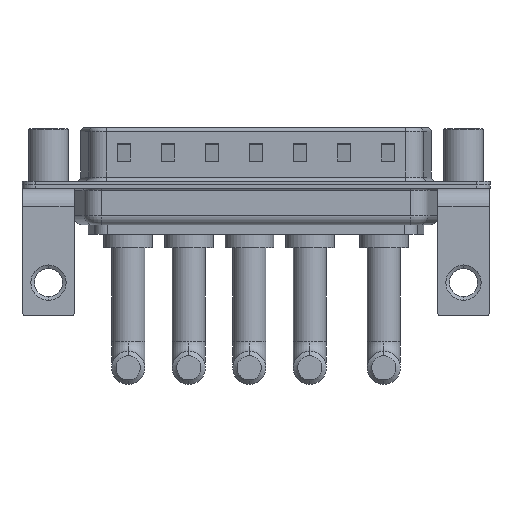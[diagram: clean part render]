
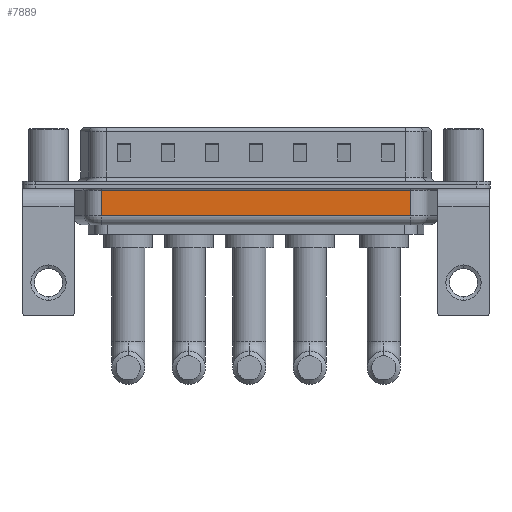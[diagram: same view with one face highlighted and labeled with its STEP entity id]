
A CAD part, front view. The second image highlights one B-rep face of the part: STEP entity #7889.
In plain terms, the highlighted planar face has unit normal (0, -1, 0).
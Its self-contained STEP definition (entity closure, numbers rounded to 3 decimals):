
#407 = EDGE_CURVE ( 'NONE', #15320, #16307, #5819, .T. ) ;
#557 = VECTOR ( 'NONE', #15797, 1000. ) ;
#854 = LINE ( 'NONE', #16324, #9173 ) ;
#1092 = PLANE ( 'NONE',  #11755 ) ;
#1909 = EDGE_LOOP ( 'NONE', ( #11771, #5399, #3220, #3569 ) ) ;
#2048 = CARTESIAN_POINT ( 'NONE',  ( 41.044, -5.35, -0.65 ) ) ;
#3220 = ORIENTED_EDGE ( 'NONE', *, *, #407, .T. ) ;
#3242 = DIRECTION ( 'NONE',  ( 0., 0., 1. ) ) ;
#3560 = VERTEX_POINT ( 'NONE', #6634 ) ;
#3569 = ORIENTED_EDGE ( 'NONE', *, *, #16784, .T. ) ;
#4444 = VERTEX_POINT ( 'NONE', #11022 ) ;
#5340 = CARTESIAN_POINT ( 'NONE',  ( 6.006, -5.35, -4.5 ) ) ;
#5399 = ORIENTED_EDGE ( 'NONE', *, *, #7920, .T. ) ;
#5819 = LINE ( 'NONE', #15003, #10045 ) ;
#6634 = CARTESIAN_POINT ( 'NONE',  ( 6.006, -5.35, -3.5 ) ) ;
#7732 = FACE_OUTER_BOUND ( 'NONE', #1909, .T. ) ;
#7889 = ADVANCED_FACE ( 'NONE', ( #7732 ), #1092, .F. ) ;
#7895 = DIRECTION ( 'NONE',  ( 0., 1., 0. ) ) ;
#7920 = EDGE_CURVE ( 'NONE', #3560, #15320, #9182, .T. ) ;
#9173 = VECTOR ( 'NONE', #11368, 1000. ) ;
#9182 = LINE ( 'NONE', #12974, #557 ) ;
#9682 = VECTOR ( 'NONE', #11806, 1000. ) ;
#9732 = CARTESIAN_POINT ( 'NONE',  ( 41.044, -5.35, -3.5 ) ) ;
#10045 = VECTOR ( 'NONE', #3242, 1000. ) ;
#11022 = CARTESIAN_POINT ( 'NONE',  ( 6.006, -5.35, -0.65 ) ) ;
#11368 = DIRECTION ( 'NONE',  ( -1., 0., 0. ) ) ;
#11755 = AXIS2_PLACEMENT_3D ( 'NONE', #5340, #7895, #12891 ) ;
#11771 = ORIENTED_EDGE ( 'NONE', *, *, #15447, .F. ) ;
#11806 = DIRECTION ( 'NONE',  ( 0., 0., 1. ) ) ;
#12891 = DIRECTION ( 'NONE',  ( 0., 0., 1. ) ) ;
#12974 = CARTESIAN_POINT ( 'NONE',  ( 6.006, -5.35, -3.5 ) ) ;
#14128 = LINE ( 'NONE', #16684, #9682 ) ;
#15003 = CARTESIAN_POINT ( 'NONE',  ( 41.044, -5.35, -4.5 ) ) ;
#15320 = VERTEX_POINT ( 'NONE', #9732 ) ;
#15447 = EDGE_CURVE ( 'NONE', #3560, #4444, #14128, .T. ) ;
#15797 = DIRECTION ( 'NONE',  ( 1., 0., 0. ) ) ;
#16307 = VERTEX_POINT ( 'NONE', #2048 ) ;
#16324 = CARTESIAN_POINT ( 'NONE',  ( 6.006, -5.35, -0.65 ) ) ;
#16684 = CARTESIAN_POINT ( 'NONE',  ( 6.006, -5.35, -4.5 ) ) ;
#16784 = EDGE_CURVE ( 'NONE', #16307, #4444, #854, .T. ) ;
